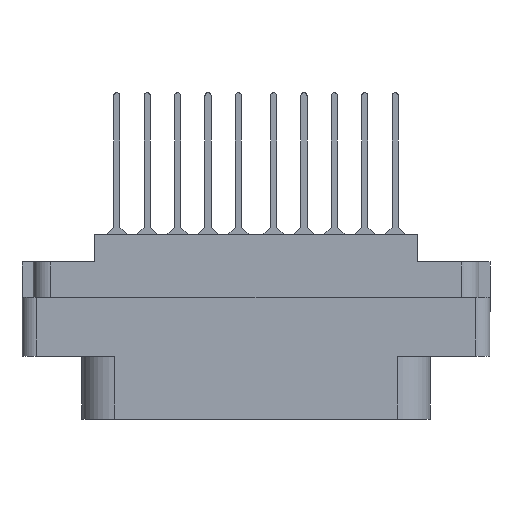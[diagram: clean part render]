
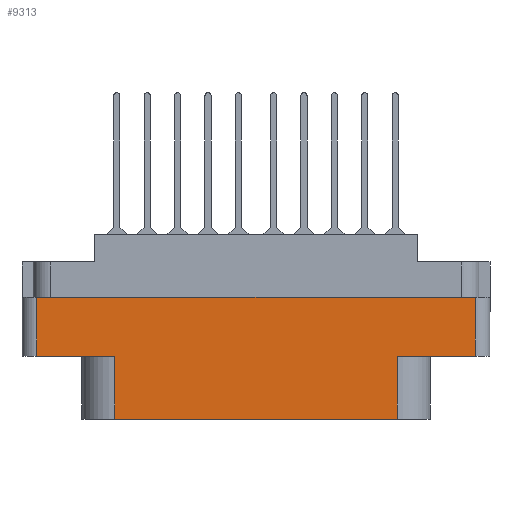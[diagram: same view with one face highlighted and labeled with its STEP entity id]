
A CAD part, front view. The second image highlights one B-rep face of the part: STEP entity #9313.
In plain terms, the highlighted planar face has unit normal (0, -1, 0).
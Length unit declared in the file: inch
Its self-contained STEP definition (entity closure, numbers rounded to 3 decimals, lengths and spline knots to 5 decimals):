
#305 = VECTOR ( 'NONE', #8341, 39.37008 ) ;
#599 = DIRECTION ( 'NONE',  ( 0., 0., -1. ) ) ;
#673 = CARTESIAN_POINT ( 'NONE',  ( -1., -0.438, -0.789 ) ) ;
#892 = DIRECTION ( 'NONE',  ( 1., 0., 0. ) ) ;
#1638 = CARTESIAN_POINT ( 'NONE',  ( 0.604, -0.438, -0.52 ) ) ;
#2249 = CARTESIAN_POINT ( 'NONE',  ( -0.938, -0.438, -0.268 ) ) ;
#2258 = EDGE_CURVE ( 'NONE', #33052, #17228, #11453, .T. ) ;
#3425 = LINE ( 'NONE', #24647, #24934 ) ;
#4664 = CARTESIAN_POINT ( 'NONE',  ( 0., -0.438, -0.52 ) ) ;
#4920 = VECTOR ( 'NONE', #26504, 39.37008 ) ;
#5115 = ORIENTED_EDGE ( 'NONE', *, *, #13788, .F. ) ;
#5295 = CARTESIAN_POINT ( 'NONE',  ( -0.604, -0.438, -0.789 ) ) ;
#5368 = CARTESIAN_POINT ( 'NONE',  ( -0.604, -0.438, -0.52 ) ) ;
#8174 = EDGE_CURVE ( 'NONE', #12225, #9872, #18339, .T. ) ;
#8181 = EDGE_CURVE ( 'NONE', #12702, #17228, #13041, .T. ) ;
#8341 = DIRECTION ( 'NONE',  ( 0., 0., -1. ) ) ;
#9313 = ADVANCED_FACE ( 'NONE', ( #28435 ), #29088, .T. ) ;
#9425 = VECTOR ( 'NONE', #18715, 39.37008 ) ;
#9429 = ORIENTED_EDGE ( 'NONE', *, *, #2258, .T. ) ;
#9872 = VERTEX_POINT ( 'NONE', #14544 ) ;
#10205 = ORIENTED_EDGE ( 'NONE', *, *, #23104, .T. ) ;
#11453 = LINE ( 'NONE', #12840, #17579 ) ;
#12225 = VERTEX_POINT ( 'NONE', #5295 ) ;
#12488 = LINE ( 'NONE', #24217, #305 ) ;
#12702 = VERTEX_POINT ( 'NONE', #2249 ) ;
#12840 = CARTESIAN_POINT ( 'NONE',  ( 0.938, -0.438, -0.789 ) ) ;
#12941 = DIRECTION ( 'NONE',  ( 1., 0., 0. ) ) ;
#13041 = LINE ( 'NONE', #18829, #23207 ) ;
#13788 = EDGE_CURVE ( 'NONE', #33052, #25767, #27242, .T. ) ;
#14544 = CARTESIAN_POINT ( 'NONE',  ( 0.604, -0.438, -0.789 ) ) ;
#15137 = ORIENTED_EDGE ( 'NONE', *, *, #27529, .T. ) ;
#15691 = DIRECTION ( 'NONE',  ( 0., -1., 0. ) ) ;
#16560 = EDGE_CURVE ( 'NONE', #16563, #21336, #24202, .T. ) ;
#16563 = VERTEX_POINT ( 'NONE', #29063 ) ;
#17228 = VERTEX_POINT ( 'NONE', #26520 ) ;
#17579 = VECTOR ( 'NONE', #26006, 39.37008 ) ;
#18145 = VECTOR ( 'NONE', #12941, 39.37008 ) ;
#18339 = LINE ( 'NONE', #673, #9425 ) ;
#18715 = DIRECTION ( 'NONE',  ( 1., 0., 0. ) ) ;
#18829 = CARTESIAN_POINT ( 'NONE',  ( 0., -0.438, -0.268 ) ) ;
#19434 = DIRECTION ( 'NONE',  ( 0., 0., 1. ) ) ;
#19972 = EDGE_CURVE ( 'NONE', #12702, #16563, #29712, .T. ) ;
#21336 = VERTEX_POINT ( 'NONE', #5368 ) ;
#21952 = VECTOR ( 'NONE', #25447, 39.37008 ) ;
#23104 = EDGE_CURVE ( 'NONE', #9872, #25767, #3425, .T. ) ;
#23207 = VECTOR ( 'NONE', #892, 39.37008 ) ;
#23425 = ORIENTED_EDGE ( 'NONE', *, *, #8181, .F. ) ;
#24142 = EDGE_LOOP ( 'NONE', ( #23425, #33339, #31533, #15137, #26074, #10205, #5115, #9429 ) ) ;
#24202 = LINE ( 'NONE', #30822, #18145 ) ;
#24217 = CARTESIAN_POINT ( 'NONE',  ( -0.604, -0.438, -0.789 ) ) ;
#24647 = CARTESIAN_POINT ( 'NONE',  ( 0.604, -0.438, -0.52 ) ) ;
#24934 = VECTOR ( 'NONE', #19434, 39.37008 ) ;
#25430 = AXIS2_PLACEMENT_3D ( 'NONE', #26357, #15691, #599 ) ;
#25447 = DIRECTION ( 'NONE',  ( -1., 0., 0. ) ) ;
#25767 = VERTEX_POINT ( 'NONE', #1638 ) ;
#26006 = DIRECTION ( 'NONE',  ( 0., 0., 1. ) ) ;
#26074 = ORIENTED_EDGE ( 'NONE', *, *, #8174, .T. ) ;
#26357 = CARTESIAN_POINT ( 'NONE',  ( -1., -0.438, -0.789 ) ) ;
#26504 = DIRECTION ( 'NONE',  ( 0., 0., -1. ) ) ;
#26520 = CARTESIAN_POINT ( 'NONE',  ( 0.938, -0.438, -0.268 ) ) ;
#27242 = LINE ( 'NONE', #4664, #21952 ) ;
#27529 = EDGE_CURVE ( 'NONE', #21336, #12225, #12488, .T. ) ;
#28435 = FACE_OUTER_BOUND ( 'NONE', #24142, .T. ) ;
#29063 = CARTESIAN_POINT ( 'NONE',  ( -0.938, -0.438, -0.52 ) ) ;
#29088 = PLANE ( 'NONE',  #25430 ) ;
#29712 = LINE ( 'NONE', #31960, #4920 ) ;
#30506 = CARTESIAN_POINT ( 'NONE',  ( 0.938, -0.438, -0.52 ) ) ;
#30822 = CARTESIAN_POINT ( 'NONE',  ( 0., -0.438, -0.52 ) ) ;
#31533 = ORIENTED_EDGE ( 'NONE', *, *, #16560, .T. ) ;
#31960 = CARTESIAN_POINT ( 'NONE',  ( -0.938, -0.438, -0.789 ) ) ;
#33052 = VERTEX_POINT ( 'NONE', #30506 ) ;
#33339 = ORIENTED_EDGE ( 'NONE', *, *, #19972, .T. ) ;
